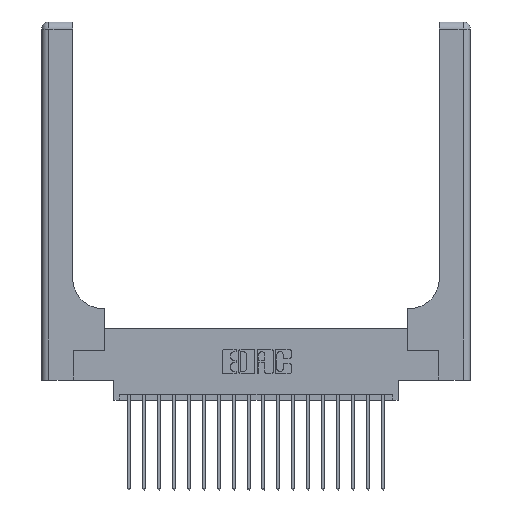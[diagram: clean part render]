
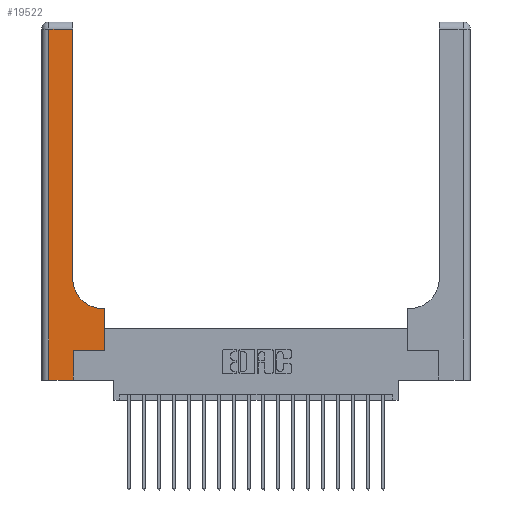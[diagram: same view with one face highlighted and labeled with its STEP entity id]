
A CAD part, top view. The second image highlights one B-rep face of the part: STEP entity #19522.
In plain terms, the highlighted planar face has unit normal (0, 0, 1).
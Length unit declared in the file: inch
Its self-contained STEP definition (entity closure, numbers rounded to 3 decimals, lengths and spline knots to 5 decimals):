
#897 = ORIENTED_EDGE ( 'NONE', *, *, #2849, .T. ) ;
#1358 = DIRECTION ( 'NONE',  ( 0., 1., 0. ) ) ;
#1374 = CARTESIAN_POINT ( 'NONE',  ( 0.528, 0.6, 0.37 ) ) ;
#1542 = DIRECTION ( 'NONE',  ( -1., 0., 0. ) ) ;
#1780 = ORIENTED_EDGE ( 'NONE', *, *, #15972, .T. ) ;
#2134 = EDGE_LOOP ( 'NONE', ( #10066, #13162, #19436, #16683, #18573, #897, #1780, #5991, #3464 ) ) ;
#2551 = VERTEX_POINT ( 'NONE', #2921 ) ;
#2849 = EDGE_CURVE ( 'NONE', #8222, #6019, #15786, .T. ) ;
#2921 = CARTESIAN_POINT ( 'NONE',  ( 0.26, 0.85, 0.37 ) ) ;
#3394 = VECTOR ( 'NONE', #14770, 39.37008 ) ;
#3464 = ORIENTED_EDGE ( 'NONE', *, *, #6960, .T. ) ;
#3895 = CARTESIAN_POINT ( 'NONE',  ( 0.06, 0., 0.37 ) ) ;
#4170 = CARTESIAN_POINT ( 'NONE',  ( 0.26, 3., 0.37 ) ) ;
#4368 = CIRCLE ( 'NONE', #7795, 0.25 ) ;
#4882 = EDGE_CURVE ( 'NONE', #12856, #8873, #14763, .T. ) ;
#5194 = CARTESIAN_POINT ( 'NONE',  ( 0., 2.94, 0.37 ) ) ;
#5233 = VERTEX_POINT ( 'NONE', #3895 ) ;
#5367 = EDGE_CURVE ( 'NONE', #9858, #5233, #10535, .T. ) ;
#5991 = ORIENTED_EDGE ( 'NONE', *, *, #4882, .T. ) ;
#6019 = VERTEX_POINT ( 'NONE', #18761 ) ;
#6076 = VECTOR ( 'NONE', #13562, 39.37008 ) ;
#6215 = VERTEX_POINT ( 'NONE', #6730 ) ;
#6730 = CARTESIAN_POINT ( 'NONE',  ( 0.265, 0., 0.37 ) ) ;
#6933 = EDGE_CURVE ( 'NONE', #8305, #9858, #16860, .T. ) ;
#6960 = EDGE_CURVE ( 'NONE', #8873, #2551, #4368, .T. ) ;
#7117 = EDGE_CURVE ( 'NONE', #2551, #8305, #13937, .T. ) ;
#7758 = DIRECTION ( 'NONE',  ( -1., 0., 0. ) ) ;
#7795 = AXIS2_PLACEMENT_3D ( 'NONE', #17803, #8438, #19344 ) ;
#7965 = FACE_OUTER_BOUND ( 'NONE', #2134, .T. ) ;
#8222 = VERTEX_POINT ( 'NONE', #14478 ) ;
#8305 = VERTEX_POINT ( 'NONE', #16376 ) ;
#8438 = DIRECTION ( 'NONE',  ( 0., 0., -1. ) ) ;
#8561 = VECTOR ( 'NONE', #11491, 39.37008 ) ;
#8873 = VERTEX_POINT ( 'NONE', #19609 ) ;
#9365 = CARTESIAN_POINT ( 'NONE',  ( 0.26, 0.6, 0.37 ) ) ;
#9858 = VERTEX_POINT ( 'NONE', #17864 ) ;
#9861 = LINE ( 'NONE', #17071, #17712 ) ;
#10066 = ORIENTED_EDGE ( 'NONE', *, *, #7117, .T. ) ;
#10535 = LINE ( 'NONE', #18263, #18390 ) ;
#11239 = LINE ( 'NONE', #13176, #3394 ) ;
#11335 = LINE ( 'NONE', #12328, #14054 ) ;
#11491 = DIRECTION ( 'NONE',  ( -1., 0., 0. ) ) ;
#12328 = CARTESIAN_POINT ( 'NONE',  ( 0.265, 0., 0.37 ) ) ;
#12586 = VECTOR ( 'NONE', #19193, 39.37008 ) ;
#12856 = VERTEX_POINT ( 'NONE', #1374 ) ;
#13162 = ORIENTED_EDGE ( 'NONE', *, *, #6933, .T. ) ;
#13176 = CARTESIAN_POINT ( 'NONE',  ( 0.528, 0.25, 0.37 ) ) ;
#13522 = EDGE_CURVE ( 'NONE', #6215, #8222, #11335, .T. ) ;
#13549 = EDGE_CURVE ( 'NONE', #5233, #6215, #9861, .T. ) ;
#13562 = DIRECTION ( 'NONE',  ( 0., 1., 0. ) ) ;
#13937 = LINE ( 'NONE', #4170, #6076 ) ;
#13991 = CARTESIAN_POINT ( 'NONE',  ( 0., 3., 0.37 ) ) ;
#14054 = VECTOR ( 'NONE', #1358, 39.37008 ) ;
#14478 = CARTESIAN_POINT ( 'NONE',  ( 0.265, 0.25, 0.37 ) ) ;
#14759 = AXIS2_PLACEMENT_3D ( 'NONE', #13991, #17120, #7758 ) ;
#14763 = LINE ( 'NONE', #9365, #18868 ) ;
#14770 = DIRECTION ( 'NONE',  ( 0., 1., 0. ) ) ;
#15556 = PLANE ( 'NONE',  #14759 ) ;
#15786 = LINE ( 'NONE', #17589, #12586 ) ;
#15972 = EDGE_CURVE ( 'NONE', #6019, #12856, #11239, .T. ) ;
#16376 = CARTESIAN_POINT ( 'NONE',  ( 0.26, 2.94, 0.37 ) ) ;
#16683 = ORIENTED_EDGE ( 'NONE', *, *, #13549, .T. ) ;
#16860 = LINE ( 'NONE', #5194, #8561 ) ;
#17071 = CARTESIAN_POINT ( 'NONE',  ( 0., 0., 0.37 ) ) ;
#17120 = DIRECTION ( 'NONE',  ( 0., 0., -1. ) ) ;
#17589 = CARTESIAN_POINT ( 'NONE',  ( 0.265, 0.25, 0.37 ) ) ;
#17712 = VECTOR ( 'NONE', #18634, 39.37008 ) ;
#17803 = CARTESIAN_POINT ( 'NONE',  ( 0.51, 0.85, 0.37 ) ) ;
#17864 = CARTESIAN_POINT ( 'NONE',  ( 0.06, 2.94, 0.37 ) ) ;
#18263 = CARTESIAN_POINT ( 'NONE',  ( 0.06, 3., 0.37 ) ) ;
#18390 = VECTOR ( 'NONE', #19806, 39.37008 ) ;
#18573 = ORIENTED_EDGE ( 'NONE', *, *, #13522, .T. ) ;
#18634 = DIRECTION ( 'NONE',  ( 1., 0., 0. ) ) ;
#18761 = CARTESIAN_POINT ( 'NONE',  ( 0.528, 0.25, 0.37 ) ) ;
#18868 = VECTOR ( 'NONE', #1542, 39.37008 ) ;
#19193 = DIRECTION ( 'NONE',  ( 1., 0., 0. ) ) ;
#19344 = DIRECTION ( 'NONE',  ( 1., 0., 0. ) ) ;
#19436 = ORIENTED_EDGE ( 'NONE', *, *, #5367, .T. ) ;
#19522 = ADVANCED_FACE ( 'NONE', ( #7965 ), #15556, .F. ) ;
#19609 = CARTESIAN_POINT ( 'NONE',  ( 0.51, 0.6, 0.37 ) ) ;
#19806 = DIRECTION ( 'NONE',  ( 0., -1., 0. ) ) ;
